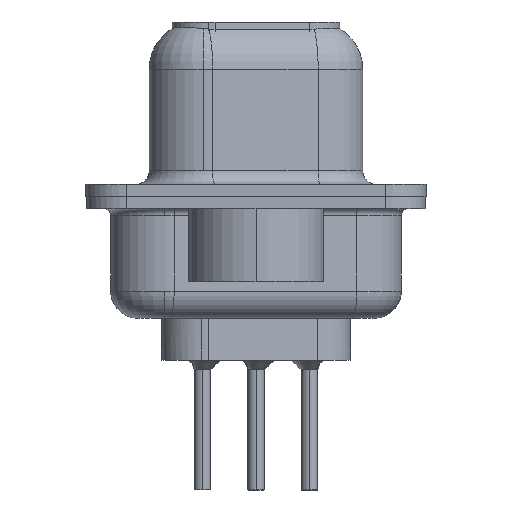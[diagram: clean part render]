
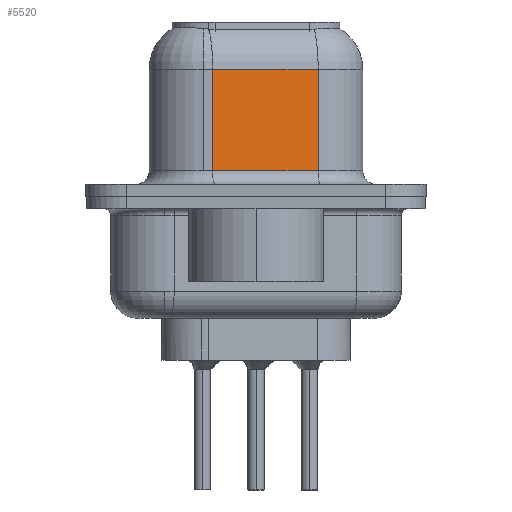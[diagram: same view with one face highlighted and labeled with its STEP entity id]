
A CAD part, left-side view. The second image highlights one B-rep face of the part: STEP entity #5520.
In plain terms, the highlighted planar face has unit normal (-0.985, -0.174, 0).
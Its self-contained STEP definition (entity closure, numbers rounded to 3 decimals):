
#369 = LINE ( 'NONE', #6584, #17252 ) ;
#735 = FACE_OUTER_BOUND ( 'NONE', #23932, .T. ) ;
#810 = DIRECTION ( 'NONE',  ( 0.985, 0.174, 0. ) ) ;
#2786 = VERTEX_POINT ( 'NONE', #18423 ) ;
#4049 = LINE ( 'NONE', #21535, #4768 ) ;
#4768 = VECTOR ( 'NONE', #23732, 1000. ) ;
#5520 = ADVANCED_FACE ( 'NONE', ( #735 ), #22838, .F. ) ;
#6488 = CARTESIAN_POINT ( 'NONE',  ( 5.063, -2.297, 6.45 ) ) ;
#6584 = CARTESIAN_POINT ( 'NONE',  ( 4.375, 1.603, 6.45 ) ) ;
#6601 = EDGE_CURVE ( 'NONE', #2786, #14140, #14509, .T. ) ;
#8329 = VECTOR ( 'NONE', #26314, 1000. ) ;
#8728 = ORIENTED_EDGE ( 'NONE', *, *, #10073, .F. ) ;
#10073 = EDGE_CURVE ( 'NONE', #2786, #16700, #14247, .T. ) ;
#14140 = VERTEX_POINT ( 'NONE', #20616 ) ;
#14247 = LINE ( 'NONE', #6488, #8329 ) ;
#14509 = LINE ( 'NONE', #15039, #19615 ) ;
#15037 = ORIENTED_EDGE ( 'NONE', *, *, #28060, .T. ) ;
#15039 = CARTESIAN_POINT ( 'NONE',  ( 5.063, -2.297, 4.7 ) ) ;
#16083 = ORIENTED_EDGE ( 'NONE', *, *, #6601, .T. ) ;
#16700 = VERTEX_POINT ( 'NONE', #20375 ) ;
#17252 = VECTOR ( 'NONE', #26431, 1000. ) ;
#18423 = CARTESIAN_POINT ( 'NONE',  ( 5.063, -2.297, 4.7 ) ) ;
#19091 = EDGE_CURVE ( 'NONE', #20617, #16700, #4049, .T. ) ;
#19391 = CARTESIAN_POINT ( 'NONE',  ( 4.375, 1.603, 0.95 ) ) ;
#19615 = VECTOR ( 'NONE', #28161, 1000. ) ;
#20375 = CARTESIAN_POINT ( 'NONE',  ( 5.063, -2.297, 0.95 ) ) ;
#20616 = CARTESIAN_POINT ( 'NONE',  ( 4.375, 1.603, 4.7 ) ) ;
#20617 = VERTEX_POINT ( 'NONE', #19391 ) ;
#20669 = CARTESIAN_POINT ( 'NONE',  ( 5.063, -2.297, 6.45 ) ) ;
#21535 = CARTESIAN_POINT ( 'NONE',  ( 5.063, -2.297, 0.95 ) ) ;
#22838 = PLANE ( 'NONE',  #24923 ) ;
#23732 = DIRECTION ( 'NONE',  ( 0.174, -0.985, 0. ) ) ;
#23932 = EDGE_LOOP ( 'NONE', ( #8728, #16083, #15037, #26667 ) ) ;
#24923 = AXIS2_PLACEMENT_3D ( 'NONE', #20669, #810, #25056 ) ;
#25056 = DIRECTION ( 'NONE',  ( -0.174, 0.985, 0. ) ) ;
#26314 = DIRECTION ( 'NONE',  ( 0., 0., -1. ) ) ;
#26431 = DIRECTION ( 'NONE',  ( 0., 0., -1. ) ) ;
#26667 = ORIENTED_EDGE ( 'NONE', *, *, #19091, .T. ) ;
#28060 = EDGE_CURVE ( 'NONE', #14140, #20617, #369, .T. ) ;
#28161 = DIRECTION ( 'NONE',  ( -0.174, 0.985, 0. ) ) ;
